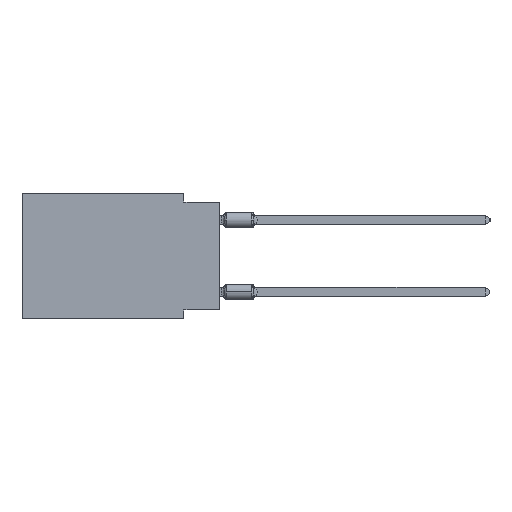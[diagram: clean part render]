
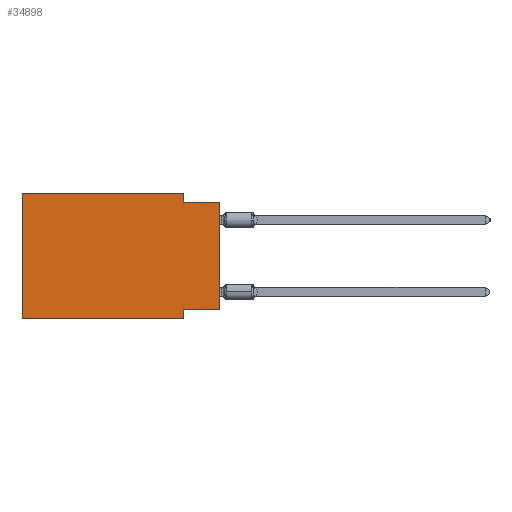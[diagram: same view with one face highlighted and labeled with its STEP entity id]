
A CAD part, left-side view. The second image highlights one B-rep face of the part: STEP entity #34898.
In plain terms, the highlighted planar face has unit normal (-1, 0, 0).
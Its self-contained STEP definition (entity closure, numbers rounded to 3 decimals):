
#347 = ORIENTED_EDGE ( 'NONE', *, *, #27642, .F. ) ;
#604 = LINE ( 'NONE', #46226, #15717 ) ;
#1348 = EDGE_LOOP ( 'NONE', ( #45150, #2950, #19933, #347, #23614, #23485, #25362, #42685 ) ) ;
#1626 = VERTEX_POINT ( 'NONE', #7859 ) ;
#1672 = PLANE ( 'NONE',  #43742 ) ;
#1830 = EDGE_CURVE ( 'NONE', #1626, #9207, #40300, .T. ) ;
#2579 = DIRECTION ( 'NONE',  ( 0., 0., -1. ) ) ;
#2950 = ORIENTED_EDGE ( 'NONE', *, *, #38038, .F. ) ;
#4655 = CARTESIAN_POINT ( 'NONE',  ( 0., 13.97, -8.89 ) ) ;
#5582 = CARTESIAN_POINT ( 'NONE',  ( 0., 0., -0.635 ) ) ;
#5900 = CARTESIAN_POINT ( 'NONE',  ( 0., 13.97, 0. ) ) ;
#7043 = EDGE_CURVE ( 'NONE', #1626, #40686, #604, .T. ) ;
#7788 = CARTESIAN_POINT ( 'NONE',  ( 0., 13.97, 0. ) ) ;
#7859 = CARTESIAN_POINT ( 'NONE',  ( 0., 0., -8.255 ) ) ;
#7925 = VECTOR ( 'NONE', #17266, 1000. ) ;
#9207 = VERTEX_POINT ( 'NONE', #14393 ) ;
#9326 = CARTESIAN_POINT ( 'NONE',  ( 0., 2.54, -8.89 ) ) ;
#11047 = CARTESIAN_POINT ( 'NONE',  ( 0., 2.54, -8.89 ) ) ;
#11406 = VERTEX_POINT ( 'NONE', #35626 ) ;
#11754 = DIRECTION ( 'NONE',  ( 0., 0., 1. ) ) ;
#14085 = DIRECTION ( 'NONE',  ( 1., 0., 0. ) ) ;
#14393 = CARTESIAN_POINT ( 'NONE',  ( 0., 0., -0.635 ) ) ;
#15604 = EDGE_CURVE ( 'NONE', #16535, #17438, #41757, .T. ) ;
#15717 = VECTOR ( 'NONE', #38314, 1000. ) ;
#16535 = VERTEX_POINT ( 'NONE', #4655 ) ;
#16593 = LINE ( 'NONE', #27075, #22876 ) ;
#17266 = DIRECTION ( 'NONE',  ( 0., 0., 1. ) ) ;
#17299 = EDGE_CURVE ( 'NONE', #16535, #19291, #38696, .T. ) ;
#17438 = VERTEX_POINT ( 'NONE', #34728 ) ;
#18553 = DIRECTION ( 'NONE',  ( 0., -1., 0. ) ) ;
#18569 = VECTOR ( 'NONE', #43516, 1000. ) ;
#19291 = VERTEX_POINT ( 'NONE', #11047 ) ;
#19865 = CARTESIAN_POINT ( 'NONE',  ( 0., 13.97, -8.89 ) ) ;
#19933 = ORIENTED_EDGE ( 'NONE', *, *, #27347, .F. ) ;
#22876 = VECTOR ( 'NONE', #24028, 1000. ) ;
#23485 = ORIENTED_EDGE ( 'NONE', *, *, #17299, .T. ) ;
#23614 = ORIENTED_EDGE ( 'NONE', *, *, #15604, .F. ) ;
#24028 = DIRECTION ( 'NONE',  ( 0., 0., -1. ) ) ;
#25362 = ORIENTED_EDGE ( 'NONE', *, *, #35305, .F. ) ;
#27075 = CARTESIAN_POINT ( 'NONE',  ( 0., 2.54, 0. ) ) ;
#27347 = EDGE_CURVE ( 'NONE', #11406, #31006, #16593, .T. ) ;
#27642 = EDGE_CURVE ( 'NONE', #17438, #11406, #29452, .T. ) ;
#29452 = LINE ( 'NONE', #45051, #45032 ) ;
#29512 = VECTOR ( 'NONE', #2579, 1000. ) ;
#30194 = VECTOR ( 'NONE', #46377, 1000. ) ;
#31006 = VERTEX_POINT ( 'NONE', #40409 ) ;
#34728 = CARTESIAN_POINT ( 'NONE',  ( 0., 13.97, 0. ) ) ;
#34898 = ADVANCED_FACE ( 'NONE', ( #48029 ), #1672, .F. ) ;
#35305 = EDGE_CURVE ( 'NONE', #40686, #19291, #36566, .T. ) ;
#35626 = CARTESIAN_POINT ( 'NONE',  ( 0., 2.54, 0. ) ) ;
#36566 = LINE ( 'NONE', #9326, #29512 ) ;
#37055 = CARTESIAN_POINT ( 'NONE',  ( 0., 2.54, -8.255 ) ) ;
#37190 = VECTOR ( 'NONE', #11754, 1000. ) ;
#38038 = EDGE_CURVE ( 'NONE', #31006, #9207, #39555, .T. ) ;
#38314 = DIRECTION ( 'NONE',  ( 0., 1., 0. ) ) ;
#38696 = LINE ( 'NONE', #19865, #30194 ) ;
#39555 = LINE ( 'NONE', #5582, #18569 ) ;
#40300 = LINE ( 'NONE', #44250, #7925 ) ;
#40409 = CARTESIAN_POINT ( 'NONE',  ( 0., 2.54, -0.635 ) ) ;
#40686 = VERTEX_POINT ( 'NONE', #37055 ) ;
#41757 = LINE ( 'NONE', #7788, #37190 ) ;
#42685 = ORIENTED_EDGE ( 'NONE', *, *, #7043, .F. ) ;
#43516 = DIRECTION ( 'NONE',  ( 0., -1., 0. ) ) ;
#43742 = AXIS2_PLACEMENT_3D ( 'NONE', #5900, #14085, #43835 ) ;
#43835 = DIRECTION ( 'NONE',  ( 0., 0., -1. ) ) ;
#44250 = CARTESIAN_POINT ( 'NONE',  ( 0., 0., 0. ) ) ;
#45032 = VECTOR ( 'NONE', #18553, 1000. ) ;
#45051 = CARTESIAN_POINT ( 'NONE',  ( 0., 13.97, 0. ) ) ;
#45150 = ORIENTED_EDGE ( 'NONE', *, *, #1830, .T. ) ;
#46226 = CARTESIAN_POINT ( 'NONE',  ( 0., 0., -8.255 ) ) ;
#46377 = DIRECTION ( 'NONE',  ( 0., -1., 0. ) ) ;
#48029 = FACE_OUTER_BOUND ( 'NONE', #1348, .T. ) ;
